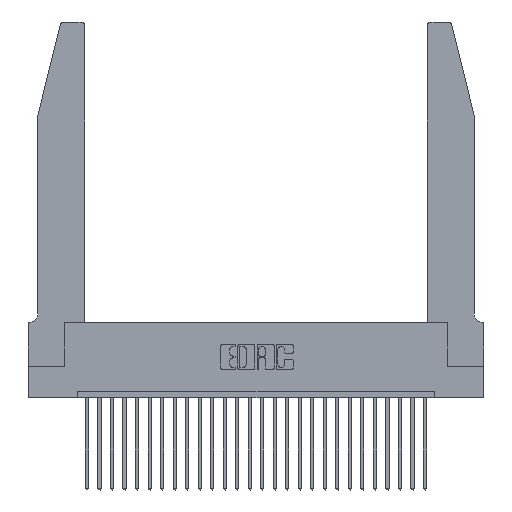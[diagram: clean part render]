
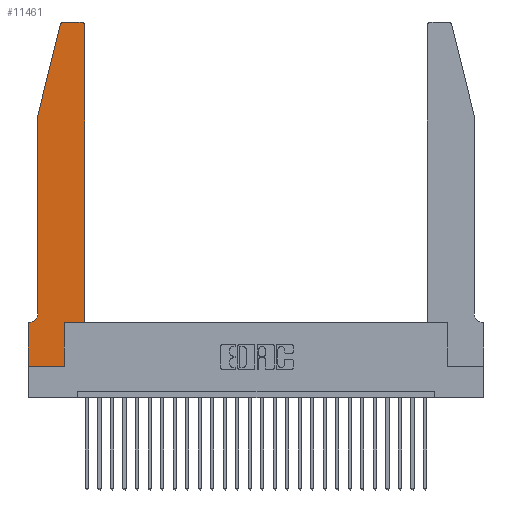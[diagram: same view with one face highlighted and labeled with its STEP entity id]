
A CAD part, top view. The second image highlights one B-rep face of the part: STEP entity #11461.
In plain terms, the highlighted planar face has unit normal (0, 0, 1).
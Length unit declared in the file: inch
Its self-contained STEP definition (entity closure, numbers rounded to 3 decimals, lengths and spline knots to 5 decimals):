
#147 = VECTOR ( 'NONE', #22463, 39.37008 ) ;
#209 = ORIENTED_EDGE ( 'NONE', *, *, #4455, .T. ) ;
#627 = DIRECTION ( 'NONE',  ( 1., 0., 0. ) ) ;
#808 = CARTESIAN_POINT ( 'NONE',  ( 0., 0.35, 0.37 ) ) ;
#921 = VECTOR ( 'NONE', #1104, 39.37008 ) ;
#1104 = DIRECTION ( 'NONE',  ( -0.239, -0.971, 0. ) ) ;
#1256 = ORIENTED_EDGE ( 'NONE', *, *, #18606, .T. ) ;
#1271 = EDGE_CURVE ( 'NONE', #26621, #4660, #14428, .T. ) ;
#1296 = VERTEX_POINT ( 'NONE', #13975 ) ;
#1493 = CARTESIAN_POINT ( 'NONE',  ( 0.284, 2.75, 0.37 ) ) ;
#2140 = EDGE_LOOP ( 'NONE', ( #1256, #24276, #27144, #209, #11449, #21787, #15161, #24085, #6885, #3388, #17654, #25007 ) ) ;
#2512 = EDGE_CURVE ( 'NONE', #11154, #24653, #13991, .T. ) ;
#3060 = DIRECTION ( 'NONE',  ( -1., 0., 0. ) ) ;
#3388 = ORIENTED_EDGE ( 'NONE', *, *, #25622, .T. ) ;
#3523 = DIRECTION ( 'NONE',  ( -1., 0., 0. ) ) ;
#4334 = DIRECTION ( 'NONE',  ( 1., 0., 0. ) ) ;
#4455 = EDGE_CURVE ( 'NONE', #24653, #19633, #11916, .T. ) ;
#4593 = VECTOR ( 'NONE', #8831, 39.37008 ) ;
#4660 = VERTEX_POINT ( 'NONE', #6162 ) ;
#4816 = LINE ( 'NONE', #22964, #18845 ) ;
#4925 = LINE ( 'NONE', #10373, #4593 ) ;
#5110 = CARTESIAN_POINT ( 'NONE',  ( 0.0755, 2., 0.37 ) ) ;
#5452 = CARTESIAN_POINT ( 'NONE',  ( 0.2865, 0.35, 0.37 ) ) ;
#5922 = CARTESIAN_POINT ( 'NONE',  ( 0.4505, 0.35, 0.37 ) ) ;
#6162 = CARTESIAN_POINT ( 'NONE',  ( 0.2865, 0., 0.37 ) ) ;
#6555 = VECTOR ( 'NONE', #23538, 39.37008 ) ;
#6885 = ORIENTED_EDGE ( 'NONE', *, *, #14709, .T. ) ;
#7148 = AXIS2_PLACEMENT_3D ( 'NONE', #15522, #19832, #627 ) ;
#7311 = CARTESIAN_POINT ( 'NONE',  ( 0.2605, 2.75, 0.37 ) ) ;
#7380 = CARTESIAN_POINT ( 'NONE',  ( 0., 0.35, 0.37 ) ) ;
#7777 = VERTEX_POINT ( 'NONE', #1493 ) ;
#7813 = DIRECTION ( 'NONE',  ( 0., 1., 0. ) ) ;
#8547 = CIRCLE ( 'NONE', #27092, 0.03 ) ;
#8575 = EDGE_CURVE ( 'NONE', #11513, #19225, #27584, .T. ) ;
#8602 = EDGE_CURVE ( 'NONE', #7777, #11154, #8547, .T. ) ;
#8688 = CARTESIAN_POINT ( 'NONE',  ( 0.25487, 2.72718, 0.37 ) ) ;
#8730 = CARTESIAN_POINT ( 'NONE',  ( 0.0755, 2., 0.37 ) ) ;
#8766 = VECTOR ( 'NONE', #10866, 39.37008 ) ;
#8831 = DIRECTION ( 'NONE',  ( -1., 0., 0. ) ) ;
#10118 = VERTEX_POINT ( 'NONE', #15422 ) ;
#10236 = CARTESIAN_POINT ( 'NONE',  ( 0.4505, 0.35, 0.37 ) ) ;
#10339 = CIRCLE ( 'NONE', #19905, 0.07 ) ;
#10373 = CARTESIAN_POINT ( 'NONE',  ( 0.0755, 0.35, 0.37 ) ) ;
#10866 = DIRECTION ( 'NONE',  ( 1., 0., 0. ) ) ;
#11154 = VERTEX_POINT ( 'NONE', #8688 ) ;
#11449 = ORIENTED_EDGE ( 'NONE', *, *, #13797, .T. ) ;
#11461 = ADVANCED_FACE ( 'NONE', ( #17422 ), #12824, .T. ) ;
#11513 = VERTEX_POINT ( 'NONE', #17941 ) ;
#11916 = LINE ( 'NONE', #8730, #6555 ) ;
#12396 = CARTESIAN_POINT ( 'NONE',  ( 0.0055, 0.42, 0.37 ) ) ;
#12623 = CIRCLE ( 'NONE', #7148, 0.03 ) ;
#12824 = PLANE ( 'NONE',  #13716 ) ;
#13716 = AXIS2_PLACEMENT_3D ( 'NONE', #7380, #27699, #4334 ) ;
#13797 = EDGE_CURVE ( 'NONE', #19633, #18902, #10339, .T. ) ;
#13975 = CARTESIAN_POINT ( 'NONE',  ( 0.2865, 0.35, 0.37 ) ) ;
#13991 = LINE ( 'NONE', #5110, #921 ) ;
#14226 = LINE ( 'NONE', #5922, #147 ) ;
#14231 = CARTESIAN_POINT ( 'NONE',  ( 0.284, 2.72, 0.37 ) ) ;
#14428 = LINE ( 'NONE', #19426, #8766 ) ;
#14709 = EDGE_CURVE ( 'NONE', #4660, #1296, #16250, .T. ) ;
#15161 = ORIENTED_EDGE ( 'NONE', *, *, #16410, .T. ) ;
#15422 = CARTESIAN_POINT ( 'NONE',  ( 0.4205, 2.75, 0.37 ) ) ;
#15522 = CARTESIAN_POINT ( 'NONE',  ( 0.4205, 2.72, 0.37 ) ) ;
#16250 = LINE ( 'NONE', #5452, #24948 ) ;
#16410 = EDGE_CURVE ( 'NONE', #19559, #26621, #4816, .T. ) ;
#16636 = CARTESIAN_POINT ( 'NONE',  ( 0.0055, 0.35, 0.37 ) ) ;
#17422 = FACE_OUTER_BOUND ( 'NONE', #2140, .T. ) ;
#17654 = ORIENTED_EDGE ( 'NONE', *, *, #8575, .T. ) ;
#17941 = CARTESIAN_POINT ( 'NONE',  ( 0.4505, 0.35, 0.37 ) ) ;
#18170 = CARTESIAN_POINT ( 'NONE',  ( 0.4505, 2.72, 0.37 ) ) ;
#18606 = EDGE_CURVE ( 'NONE', #10118, #7777, #21485, .T. ) ;
#18845 = VECTOR ( 'NONE', #27452, 39.37008 ) ;
#18899 = VECTOR ( 'NONE', #7813, 39.37008 ) ;
#18902 = VERTEX_POINT ( 'NONE', #16636 ) ;
#18967 = CARTESIAN_POINT ( 'NONE',  ( 0.0755, 0.42, 0.37 ) ) ;
#19225 = VERTEX_POINT ( 'NONE', #18170 ) ;
#19426 = CARTESIAN_POINT ( 'NONE',  ( 0., 0., 0.37 ) ) ;
#19559 = VERTEX_POINT ( 'NONE', #808 ) ;
#19633 = VERTEX_POINT ( 'NONE', #18967 ) ;
#19832 = DIRECTION ( 'NONE',  ( 0., 0., 1. ) ) ;
#19905 = AXIS2_PLACEMENT_3D ( 'NONE', #12396, #27344, #3523 ) ;
#21485 = LINE ( 'NONE', #7311, #26823 ) ;
#21787 = ORIENTED_EDGE ( 'NONE', *, *, #24972, .T. ) ;
#22045 = EDGE_CURVE ( 'NONE', #19225, #10118, #12623, .T. ) ;
#22463 = DIRECTION ( 'NONE',  ( 1., 0., 0. ) ) ;
#22594 = CARTESIAN_POINT ( 'NONE',  ( 0., 0., 0.37 ) ) ;
#22964 = CARTESIAN_POINT ( 'NONE',  ( 0., 0., 0.37 ) ) ;
#22978 = DIRECTION ( 'NONE',  ( 0., 1., 0. ) ) ;
#23538 = DIRECTION ( 'NONE',  ( 0., -1., 0. ) ) ;
#24085 = ORIENTED_EDGE ( 'NONE', *, *, #1271, .T. ) ;
#24276 = ORIENTED_EDGE ( 'NONE', *, *, #8602, .T. ) ;
#24653 = VERTEX_POINT ( 'NONE', #26452 ) ;
#24948 = VECTOR ( 'NONE', #22978, 39.37008 ) ;
#24972 = EDGE_CURVE ( 'NONE', #18902, #19559, #4925, .T. ) ;
#24973 = DIRECTION ( 'NONE',  ( 0., 0., 1. ) ) ;
#25007 = ORIENTED_EDGE ( 'NONE', *, *, #22045, .T. ) ;
#25622 = EDGE_CURVE ( 'NONE', #1296, #11513, #14226, .T. ) ;
#26452 = CARTESIAN_POINT ( 'NONE',  ( 0.0755, 2., 0.37 ) ) ;
#26621 = VERTEX_POINT ( 'NONE', #22594 ) ;
#26823 = VECTOR ( 'NONE', #3060, 39.37008 ) ;
#27092 = AXIS2_PLACEMENT_3D ( 'NONE', #14231, #24973, #27209 ) ;
#27144 = ORIENTED_EDGE ( 'NONE', *, *, #2512, .T. ) ;
#27209 = DIRECTION ( 'NONE',  ( 1., 0., 0. ) ) ;
#27344 = DIRECTION ( 'NONE',  ( 0., 0., -1. ) ) ;
#27452 = DIRECTION ( 'NONE',  ( 0., -1., 0. ) ) ;
#27584 = LINE ( 'NONE', #10236, #18899 ) ;
#27699 = DIRECTION ( 'NONE',  ( 0., 0., 1. ) ) ;
